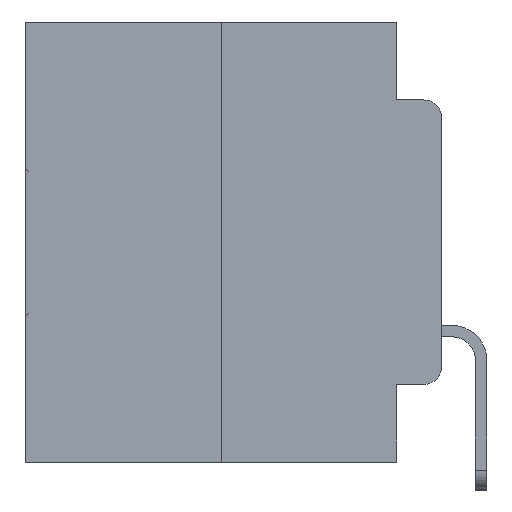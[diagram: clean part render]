
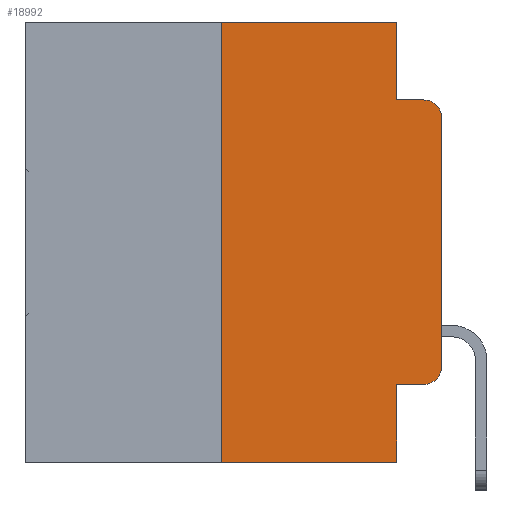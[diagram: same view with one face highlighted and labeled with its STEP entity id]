
A CAD part, left-side view. The second image highlights one B-rep face of the part: STEP entity #18992.
In plain terms, the highlighted planar face has unit normal (-1, 0, 0).
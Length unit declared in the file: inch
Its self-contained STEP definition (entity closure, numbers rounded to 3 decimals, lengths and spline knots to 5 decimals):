
#284 = DIRECTION ( 'NONE',  ( 0., -1., 0. ) ) ;
#371 = CARTESIAN_POINT ( 'NONE',  ( 0., 0.25, 0. ) ) ;
#552 = DIRECTION ( 'NONE',  ( 0., 0., -1. ) ) ;
#777 = VERTEX_POINT ( 'NONE', #22292 ) ;
#875 = EDGE_CURVE ( 'NONE', #27468, #19692, #12987, .T. ) ;
#1232 = ORIENTED_EDGE ( 'NONE', *, *, #24344, .F. ) ;
#1459 = ORIENTED_EDGE ( 'NONE', *, *, #8754, .T. ) ;
#1660 = DIRECTION ( 'NONE',  ( 0., -1., 0. ) ) ;
#3221 = CARTESIAN_POINT ( 'NONE',  ( 0., 0.02, -0.0885 ) ) ;
#3572 = DIRECTION ( 'NONE',  ( -1., 0., 0. ) ) ;
#5266 = LINE ( 'NONE', #371, #16791 ) ;
#5411 = CARTESIAN_POINT ( 'NONE',  ( 0., 0., -0.1085 ) ) ;
#5779 = LINE ( 'NONE', #20901, #28930 ) ;
#6700 = VERTEX_POINT ( 'NONE', #3221 ) ;
#6887 = CARTESIAN_POINT ( 'NONE',  ( 0., 0.473, 0. ) ) ;
#7037 = DIRECTION ( 'NONE',  ( -1., 0., 0. ) ) ;
#7038 = ORIENTED_EDGE ( 'NONE', *, *, #9551, .T. ) ;
#7185 = EDGE_CURVE ( 'NONE', #19692, #6700, #5779, .T. ) ;
#7480 = ORIENTED_EDGE ( 'NONE', *, *, #17794, .F. ) ;
#8214 = ORIENTED_EDGE ( 'NONE', *, *, #16975, .T. ) ;
#8396 = VECTOR ( 'NONE', #15737, 39.37008 ) ;
#8754 = EDGE_CURVE ( 'NONE', #20155, #6700, #12933, .T. ) ;
#8837 = VERTEX_POINT ( 'NONE', #28489 ) ;
#9551 = EDGE_CURVE ( 'NONE', #9796, #777, #23397, .T. ) ;
#9770 = CARTESIAN_POINT ( 'NONE',  ( 0., 0.051, 0. ) ) ;
#9796 = VERTEX_POINT ( 'NONE', #25101 ) ;
#10006 = CARTESIAN_POINT ( 'NONE',  ( 0., 0.051, 0. ) ) ;
#10115 = CIRCLE ( 'NONE', #10792, 0.02 ) ;
#10583 = VECTOR ( 'NONE', #13593, 39.37008 ) ;
#10706 = VECTOR ( 'NONE', #25398, 39.37008 ) ;
#10782 = VECTOR ( 'NONE', #1660, 39.37008 ) ;
#10792 = AXIS2_PLACEMENT_3D ( 'NONE', #20659, #7037, #22848 ) ;
#11541 = PLANE ( 'NONE',  #26944 ) ;
#11581 = EDGE_LOOP ( 'NONE', ( #15635, #1459, #20829, #22000, #7480, #1232, #7038, #23772, #8214, #19651 ) ) ;
#12305 = CARTESIAN_POINT ( 'NONE',  ( 0., 0.051, -0.0885 ) ) ;
#12400 = EDGE_CURVE ( 'NONE', #29308, #8837, #10115, .T. ) ;
#12933 = CIRCLE ( 'NONE', #24685, 0.02 ) ;
#12987 = LINE ( 'NONE', #10006, #18294 ) ;
#13262 = CARTESIAN_POINT ( 'NONE',  ( 0., 0.473, -0.5 ) ) ;
#13456 = CARTESIAN_POINT ( 'NONE',  ( 0., 0.051, -0.4115 ) ) ;
#13503 = CARTESIAN_POINT ( 'NONE',  ( 0., 0.02, -0.4115 ) ) ;
#13593 = DIRECTION ( 'NONE',  ( 0., 0., 1. ) ) ;
#13839 = DIRECTION ( 'NONE',  ( 1., 0., 0. ) ) ;
#14323 = DIRECTION ( 'NONE',  ( 0., 0., 1. ) ) ;
#15609 = CARTESIAN_POINT ( 'NONE',  ( 0., 0.051, 0. ) ) ;
#15635 = ORIENTED_EDGE ( 'NONE', *, *, #16414, .T. ) ;
#15737 = DIRECTION ( 'NONE',  ( 0., -1., 0. ) ) ;
#16414 = EDGE_CURVE ( 'NONE', #8837, #20155, #28324, .T. ) ;
#16791 = VECTOR ( 'NONE', #14323, 39.37008 ) ;
#16975 = EDGE_CURVE ( 'NONE', #20545, #29308, #20445, .T. ) ;
#17380 = CARTESIAN_POINT ( 'NONE',  ( 0., 0.02, -0.1085 ) ) ;
#17537 = VERTEX_POINT ( 'NONE', #22128 ) ;
#17794 = EDGE_CURVE ( 'NONE', #17537, #27468, #23020, .T. ) ;
#18294 = VECTOR ( 'NONE', #552, 39.37008 ) ;
#18472 = EDGE_CURVE ( 'NONE', #20545, #777, #21961, .T. ) ;
#18992 = ADVANCED_FACE ( 'NONE', ( #24997 ), #11541, .F. ) ;
#19601 = DIRECTION ( 'NONE',  ( 0., 0., -1. ) ) ;
#19651 = ORIENTED_EDGE ( 'NONE', *, *, #12400, .T. ) ;
#19692 = VERTEX_POINT ( 'NONE', #12305 ) ;
#20155 = VERTEX_POINT ( 'NONE', #5411 ) ;
#20279 = CARTESIAN_POINT ( 'NONE',  ( 0., 0., 0. ) ) ;
#20445 = LINE ( 'NONE', #13456, #8396 ) ;
#20545 = VERTEX_POINT ( 'NONE', #22735 ) ;
#20659 = CARTESIAN_POINT ( 'NONE',  ( 0., 0.02, -0.3915 ) ) ;
#20829 = ORIENTED_EDGE ( 'NONE', *, *, #7185, .F. ) ;
#20901 = CARTESIAN_POINT ( 'NONE',  ( 0., 0.051, -0.0885 ) ) ;
#21961 = LINE ( 'NONE', #9770, #10706 ) ;
#22000 = ORIENTED_EDGE ( 'NONE', *, *, #875, .F. ) ;
#22128 = CARTESIAN_POINT ( 'NONE',  ( 0., 0.25, 0. ) ) ;
#22292 = CARTESIAN_POINT ( 'NONE',  ( 0., 0.051, -0.5 ) ) ;
#22735 = CARTESIAN_POINT ( 'NONE',  ( 0., 0.051, -0.4115 ) ) ;
#22848 = DIRECTION ( 'NONE',  ( 0., 0., -1. ) ) ;
#23020 = LINE ( 'NONE', #25247, #28141 ) ;
#23397 = LINE ( 'NONE', #13262, #10782 ) ;
#23772 = ORIENTED_EDGE ( 'NONE', *, *, #18472, .F. ) ;
#24344 = EDGE_CURVE ( 'NONE', #9796, #17537, #5266, .T. ) ;
#24685 = AXIS2_PLACEMENT_3D ( 'NONE', #17380, #3572, #19601 ) ;
#24997 = FACE_OUTER_BOUND ( 'NONE', #11581, .T. ) ;
#25101 = CARTESIAN_POINT ( 'NONE',  ( 0., 0.25, -0.5 ) ) ;
#25247 = CARTESIAN_POINT ( 'NONE',  ( 0., 0.473, 0. ) ) ;
#25398 = DIRECTION ( 'NONE',  ( 0., 0., -1. ) ) ;
#26944 = AXIS2_PLACEMENT_3D ( 'NONE', #6887, #13839, #29273 ) ;
#27447 = DIRECTION ( 'NONE',  ( 0., -1., 0. ) ) ;
#27468 = VERTEX_POINT ( 'NONE', #15609 ) ;
#28141 = VECTOR ( 'NONE', #27447, 39.37008 ) ;
#28324 = LINE ( 'NONE', #20279, #10583 ) ;
#28489 = CARTESIAN_POINT ( 'NONE',  ( 0., 0., -0.3915 ) ) ;
#28930 = VECTOR ( 'NONE', #284, 39.37008 ) ;
#29273 = DIRECTION ( 'NONE',  ( 0., 0., -1. ) ) ;
#29308 = VERTEX_POINT ( 'NONE', #13503 ) ;
